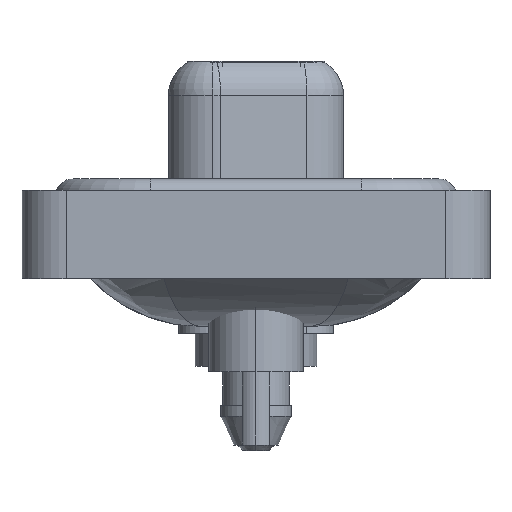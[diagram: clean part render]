
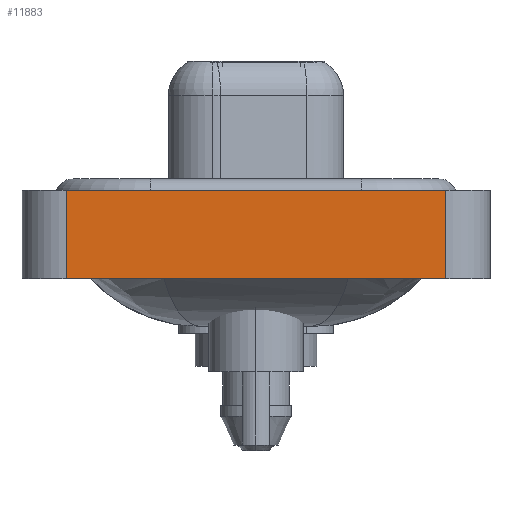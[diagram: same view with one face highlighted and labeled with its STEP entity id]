
A CAD part, left-side view. The second image highlights one B-rep face of the part: STEP entity #11883.
In plain terms, the highlighted planar face has unit normal (-1, 0, 0).
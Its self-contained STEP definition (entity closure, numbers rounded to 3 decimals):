
#558 = CARTESIAN_POINT ( 'NONE',  ( -7.35, 8.55, 0.4 ) ) ;
#608 = CARTESIAN_POINT ( 'NONE',  ( -7.35, 8.55, -3.6 ) ) ;
#666 = VECTOR ( 'NONE', #5119, 1000. ) ;
#954 = PLANE ( 'NONE',  #2080 ) ;
#1576 = CARTESIAN_POINT ( 'NONE',  ( -7.35, -8.55, -3.6 ) ) ;
#2080 = AXIS2_PLACEMENT_3D ( 'NONE', #6501, #7794, #11814 ) ;
#2202 = ORIENTED_EDGE ( 'NONE', *, *, #12205, .F. ) ;
#3171 = VERTEX_POINT ( 'NONE', #558 ) ;
#3506 = LINE ( 'NONE', #8956, #9367 ) ;
#3791 = VERTEX_POINT ( 'NONE', #1576 ) ;
#3936 = CARTESIAN_POINT ( 'NONE',  ( -7.35, -8.55, 0.4 ) ) ;
#4920 = VERTEX_POINT ( 'NONE', #608 ) ;
#5119 = DIRECTION ( 'NONE',  ( 0., -1., 0. ) ) ;
#5709 = CARTESIAN_POINT ( 'NONE',  ( -7.35, -8.55, -3.6 ) ) ;
#6501 = CARTESIAN_POINT ( 'NONE',  ( -7.35, -8.55, -3.6 ) ) ;
#7170 = LINE ( 'NONE', #5709, #9381 ) ;
#7207 = EDGE_CURVE ( 'NONE', #4920, #3791, #17168, .T. ) ;
#7794 = DIRECTION ( 'NONE',  ( -1., 0., 0. ) ) ;
#7890 = ORIENTED_EDGE ( 'NONE', *, *, #7207, .T. ) ;
#8956 = CARTESIAN_POINT ( 'NONE',  ( -7.35, 8.55, -3.6 ) ) ;
#9367 = VECTOR ( 'NONE', #15798, 1000. ) ;
#9381 = VECTOR ( 'NONE', #12916, 1000. ) ;
#10219 = CARTESIAN_POINT ( 'NONE',  ( -7.35, -8.55, -3.6 ) ) ;
#10757 = LINE ( 'NONE', #3936, #666 ) ;
#11034 = ORIENTED_EDGE ( 'NONE', *, *, #11269, .T. ) ;
#11269 = EDGE_CURVE ( 'NONE', #3791, #13820, #7170, .T. ) ;
#11814 = DIRECTION ( 'NONE',  ( 0., 0., 1. ) ) ;
#11883 = ADVANCED_FACE ( 'NONE', ( #13432 ), #954, .T. ) ;
#12205 = EDGE_CURVE ( 'NONE', #4920, #3171, #3506, .T. ) ;
#12768 = DIRECTION ( 'NONE',  ( 0., -1., 0. ) ) ;
#12916 = DIRECTION ( 'NONE',  ( 0., 0., 1. ) ) ;
#13179 = ORIENTED_EDGE ( 'NONE', *, *, #14181, .F. ) ;
#13432 = FACE_OUTER_BOUND ( 'NONE', #13925, .T. ) ;
#13820 = VERTEX_POINT ( 'NONE', #15686 ) ;
#13925 = EDGE_LOOP ( 'NONE', ( #11034, #13179, #2202, #7890 ) ) ;
#14072 = VECTOR ( 'NONE', #12768, 1000. ) ;
#14181 = EDGE_CURVE ( 'NONE', #3171, #13820, #10757, .T. ) ;
#15686 = CARTESIAN_POINT ( 'NONE',  ( -7.35, -8.55, 0.4 ) ) ;
#15798 = DIRECTION ( 'NONE',  ( 0., 0., 1. ) ) ;
#17168 = LINE ( 'NONE', #10219, #14072 ) ;
